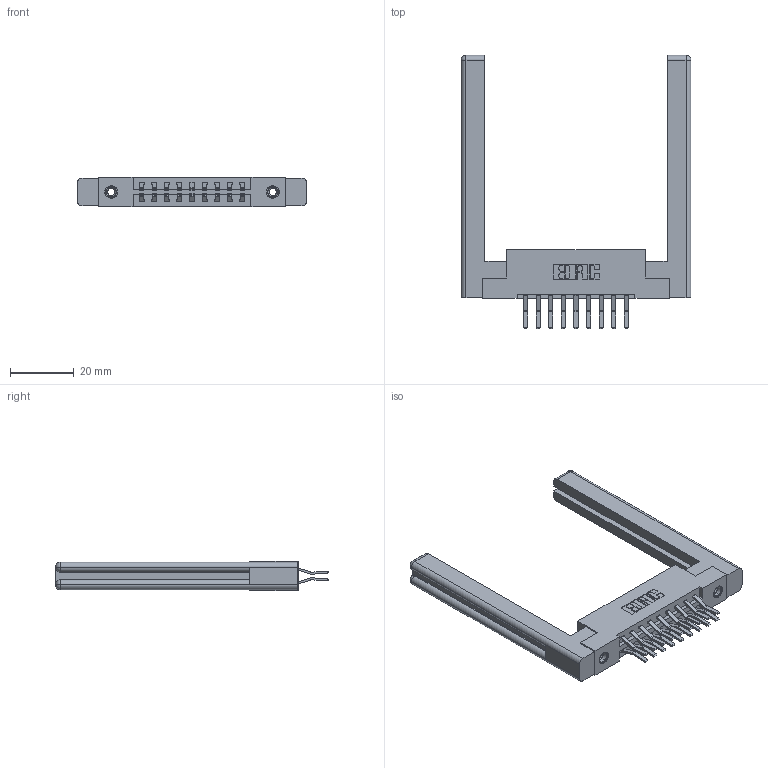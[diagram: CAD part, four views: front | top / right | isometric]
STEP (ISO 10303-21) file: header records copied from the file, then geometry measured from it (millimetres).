
FILE_DESCRIPTION (( 'STEP AP203' ), '1' );
FILE_NAME ('337-018-560-258.STEP', '2019-10-08T13:38:41', ( '' ), ( '' ), 'SwSTEP 2.0', 'SolidWorks 2016', '' );
FILE_SCHEMA (( 'CONFIG_CONTROL_DESIGN' ));
Length unit declared in the file: inch
Products named in the file (5): 337-018-560-258; 307-220-058; 345-250-001_345-250-001-102; 345-292-001_560 Tail; 337 Part_Flush Mounting Lugs - 0.156 Dia-TI
Assembly tree (23 placements, depth 2):
  337-018-560-258
    337 Part_Flush Mounting Lugs - 0.156 Dia-TI
    345-292-001_560 Tail  x18
    345-250-001_345-250-001-102  x2
    307-220-058  x2
Bounding box: 72.29 x 85.87 x 9.4 mm (x, y, z)
Volume: 14439.4 mm3; surface area: 13317 mm2
Topology: 23 solids, 23 shells, 1264 faces, 3671 edges, 2410 vertices
Faces by surface type: plane 838, cylinder 402, cone 12, torus 12
Entity records: 13968 total; most frequent: CARTESIAN_POINT 2389, ORIENTED_EDGE 2264, DIRECTION 2112, EDGE_CURVE 1132, VECTOR 952, LINE 952, VERTEX_POINT 746, AXIS2_PLACEMENT_3D 580
